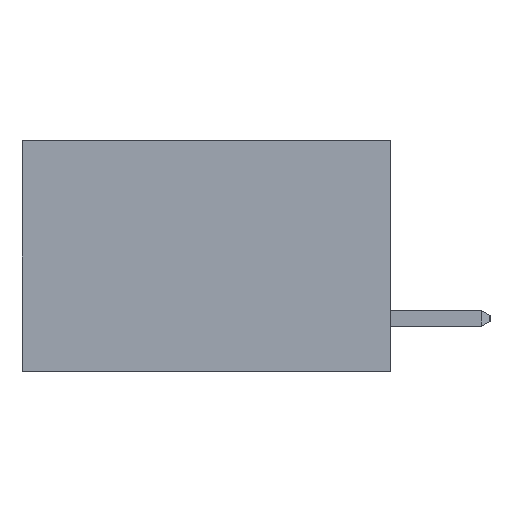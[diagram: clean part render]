
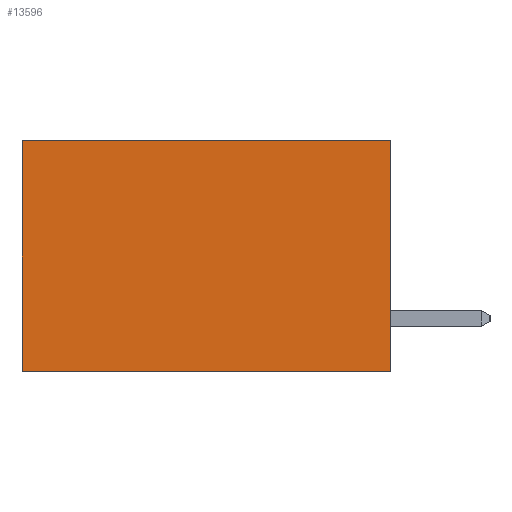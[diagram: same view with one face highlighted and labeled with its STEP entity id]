
A CAD part, left-side view. The second image highlights one B-rep face of the part: STEP entity #13596.
In plain terms, the highlighted planar face has unit normal (-1, 0, 0).
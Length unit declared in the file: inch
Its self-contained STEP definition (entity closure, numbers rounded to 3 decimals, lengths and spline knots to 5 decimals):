
#26 = CARTESIAN_POINT ( 'NONE',  ( 0.277, 0., -0.37 ) ) ;
#1520 = DIRECTION ( 'NONE',  ( 1., 0., 0. ) ) ;
#2987 = EDGE_CURVE ( 'NONE', #6324, #9369, #8947, .T. ) ;
#3254 = EDGE_CURVE ( 'NONE', #9369, #8797, #13758, .T. ) ;
#3577 = AXIS2_PLACEMENT_3D ( 'NONE', #26, #1520, #10987 ) ;
#3640 = ORIENTED_EDGE ( 'NONE', *, *, #4878, .F. ) ;
#4457 = PLANE ( 'NONE',  #3577 ) ;
#4835 = LINE ( 'NONE', #7499, #10532 ) ;
#4878 = EDGE_CURVE ( 'NONE', #6324, #5621, #4835, .T. ) ;
#4974 = CARTESIAN_POINT ( 'NONE',  ( 0.277, 0., 0. ) ) ;
#5013 = CARTESIAN_POINT ( 'NONE',  ( 0.277, 0.59, -0.37 ) ) ;
#5248 = LINE ( 'NONE', #14126, #8308 ) ;
#5400 = EDGE_CURVE ( 'NONE', #5621, #8797, #5248, .T. ) ;
#5621 = VERTEX_POINT ( 'NONE', #11392 ) ;
#5926 = CARTESIAN_POINT ( 'NONE',  ( 0.277, 0.59, 0. ) ) ;
#5944 = VECTOR ( 'NONE', #12454, 39.37008 ) ;
#6324 = VERTEX_POINT ( 'NONE', #4974 ) ;
#7259 = ORIENTED_EDGE ( 'NONE', *, *, #2987, .T. ) ;
#7499 = CARTESIAN_POINT ( 'NONE',  ( 0.277, 0., -0.37 ) ) ;
#7774 = DIRECTION ( 'NONE',  ( 0., 0., -1. ) ) ;
#8096 = CARTESIAN_POINT ( 'NONE',  ( 0.277, 0.59, -0.37 ) ) ;
#8308 = VECTOR ( 'NONE', #14109, 39.37008 ) ;
#8797 = VERTEX_POINT ( 'NONE', #5013 ) ;
#8947 = LINE ( 'NONE', #12337, #5944 ) ;
#9369 = VERTEX_POINT ( 'NONE', #5926 ) ;
#9809 = DIRECTION ( 'NONE',  ( 0., 0., -1. ) ) ;
#10417 = VECTOR ( 'NONE', #9809, 39.37008 ) ;
#10532 = VECTOR ( 'NONE', #7774, 39.37008 ) ;
#10987 = DIRECTION ( 'NONE',  ( 0., 0., -1. ) ) ;
#11392 = CARTESIAN_POINT ( 'NONE',  ( 0.277, 0., -0.37 ) ) ;
#12337 = CARTESIAN_POINT ( 'NONE',  ( 0.277, 0., 0. ) ) ;
#12454 = DIRECTION ( 'NONE',  ( 0., 1., 0. ) ) ;
#13596 = ADVANCED_FACE ( 'NONE', ( #16777 ), #4457, .F. ) ;
#13758 = LINE ( 'NONE', #8096, #10417 ) ;
#14109 = DIRECTION ( 'NONE',  ( 0., 1., 0. ) ) ;
#14126 = CARTESIAN_POINT ( 'NONE',  ( 0.277, 0., -0.37 ) ) ;
#16043 = EDGE_LOOP ( 'NONE', ( #16096, #16481, #3640, #7259 ) ) ;
#16096 = ORIENTED_EDGE ( 'NONE', *, *, #3254, .T. ) ;
#16481 = ORIENTED_EDGE ( 'NONE', *, *, #5400, .F. ) ;
#16777 = FACE_OUTER_BOUND ( 'NONE', #16043, .T. ) ;
